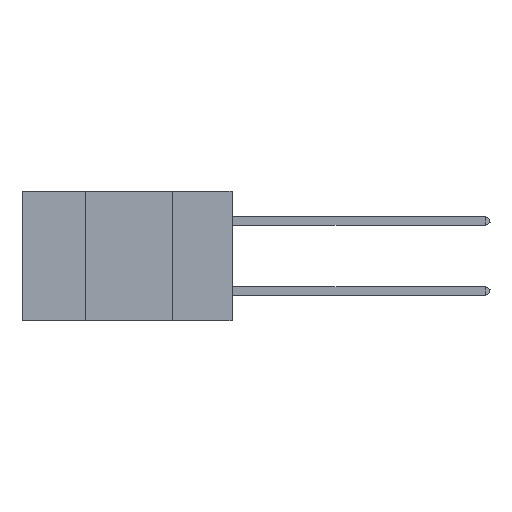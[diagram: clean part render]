
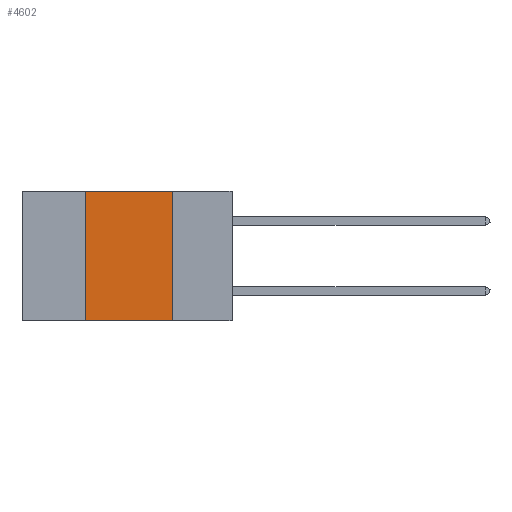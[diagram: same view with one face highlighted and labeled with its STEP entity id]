
A CAD part, left-side view. The second image highlights one B-rep face of the part: STEP entity #4602.
In plain terms, the highlighted planar face has unit normal (-1, 0, 0).
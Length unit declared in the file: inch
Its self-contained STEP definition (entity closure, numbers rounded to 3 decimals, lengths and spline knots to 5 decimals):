
#585 = VERTEX_POINT ( 'NONE', #8808 ) ;
#974 = CARTESIAN_POINT ( 'NONE',  ( 0., 0.42, 0. ) ) ;
#1127 = CARTESIAN_POINT ( 'NONE',  ( 0., 0.17, 0. ) ) ;
#1207 = DIRECTION ( 'NONE',  ( 1., 0., 0. ) ) ;
#1678 = VERTEX_POINT ( 'NONE', #1127 ) ;
#1971 = EDGE_CURVE ( 'NONE', #6001, #585, #8545, .T. ) ;
#2055 = LINE ( 'NONE', #6040, #8800 ) ;
#2100 = VECTOR ( 'NONE', #5138, 39.37008 ) ;
#2514 = DIRECTION ( 'NONE',  ( 0., 0., -1. ) ) ;
#3408 = CARTESIAN_POINT ( 'NONE',  ( 0., 0.17, 0. ) ) ;
#3413 = DIRECTION ( 'NONE',  ( 0., -1., 0. ) ) ;
#4128 = ORIENTED_EDGE ( 'NONE', *, *, #7273, .F. ) ;
#4602 = ADVANCED_FACE ( 'NONE', ( #9726 ), #5641, .F. ) ;
#4618 = AXIS2_PLACEMENT_3D ( 'NONE', #4762, #1207, #7368 ) ;
#4760 = LINE ( 'NONE', #6826, #2100 ) ;
#4762 = CARTESIAN_POINT ( 'NONE',  ( 0., 0.6, 0. ) ) ;
#4931 = VECTOR ( 'NONE', #2514, 39.37008 ) ;
#5138 = DIRECTION ( 'NONE',  ( 0., 0., 1. ) ) ;
#5641 = PLANE ( 'NONE',  #4618 ) ;
#6001 = VERTEX_POINT ( 'NONE', #8485 ) ;
#6040 = CARTESIAN_POINT ( 'NONE',  ( 0., 0.6, 0. ) ) ;
#6443 = ORIENTED_EDGE ( 'NONE', *, *, #10980, .F. ) ;
#6826 = CARTESIAN_POINT ( 'NONE',  ( 0., 0.42, 0. ) ) ;
#7229 = LINE ( 'NONE', #3408, #4931 ) ;
#7273 = EDGE_CURVE ( 'NONE', #8087, #1678, #2055, .T. ) ;
#7368 = DIRECTION ( 'NONE',  ( 0., 0., -1. ) ) ;
#7530 = CARTESIAN_POINT ( 'NONE',  ( 0., 0.6, -0.37 ) ) ;
#8087 = VERTEX_POINT ( 'NONE', #974 ) ;
#8472 = ORIENTED_EDGE ( 'NONE', *, *, #9823, .F. ) ;
#8485 = CARTESIAN_POINT ( 'NONE',  ( 0., 0.42, -0.37 ) ) ;
#8545 = LINE ( 'NONE', #7530, #10577 ) ;
#8800 = VECTOR ( 'NONE', #3413, 39.37008 ) ;
#8808 = CARTESIAN_POINT ( 'NONE',  ( 0., 0.17, -0.37 ) ) ;
#8916 = DIRECTION ( 'NONE',  ( 0., -1., 0. ) ) ;
#9035 = ORIENTED_EDGE ( 'NONE', *, *, #1971, .T. ) ;
#9726 = FACE_OUTER_BOUND ( 'NONE', #10472, .T. ) ;
#9823 = EDGE_CURVE ( 'NONE', #1678, #585, #7229, .T. ) ;
#10472 = EDGE_LOOP ( 'NONE', ( #8472, #4128, #6443, #9035 ) ) ;
#10577 = VECTOR ( 'NONE', #8916, 39.37008 ) ;
#10980 = EDGE_CURVE ( 'NONE', #6001, #8087, #4760, .T. ) ;
